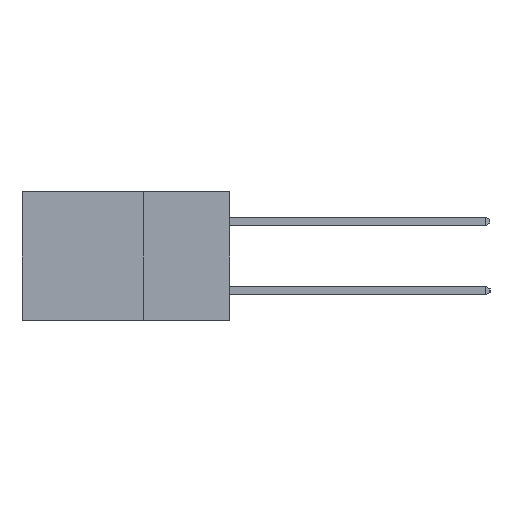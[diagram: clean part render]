
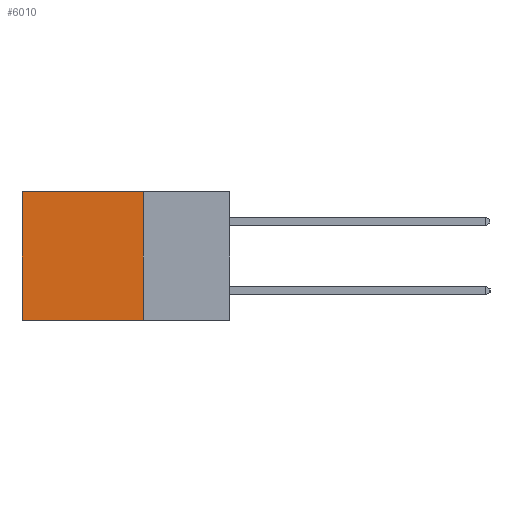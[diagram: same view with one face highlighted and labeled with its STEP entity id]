
A CAD part, left-side view. The second image highlights one B-rep face of the part: STEP entity #6010.
In plain terms, the highlighted planar face has unit normal (-1, 0, 0).
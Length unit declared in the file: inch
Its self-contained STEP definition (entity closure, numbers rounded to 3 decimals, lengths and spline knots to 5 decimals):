
#1495 = ORIENTED_EDGE ( 'NONE', *, *, #3555, .T. ) ;
#1730 = DIRECTION ( 'NONE',  ( 0., 0., -1. ) ) ;
#1794 = CARTESIAN_POINT ( 'NONE',  ( 0.2615, 0.6, -0.37 ) ) ;
#2799 = DIRECTION ( 'NONE',  ( 0., 1., 0. ) ) ;
#2877 = CARTESIAN_POINT ( 'NONE',  ( 0.2615, 0.25, -0.37 ) ) ;
#3468 = EDGE_CURVE ( 'NONE', #6410, #3936, #7399, .T. ) ;
#3555 = EDGE_CURVE ( 'NONE', #5289, #3936, #5964, .T. ) ;
#3936 = VERTEX_POINT ( 'NONE', #13215 ) ;
#4170 = CARTESIAN_POINT ( 'NONE',  ( 0.2615, 0.25, 0. ) ) ;
#5289 = VERTEX_POINT ( 'NONE', #14054 ) ;
#5964 = LINE ( 'NONE', #1794, #14185 ) ;
#6010 = ADVANCED_FACE ( 'NONE', ( #9214 ), #10509, .F. ) ;
#6410 = VERTEX_POINT ( 'NONE', #8083 ) ;
#7280 = VERTEX_POINT ( 'NONE', #4170 ) ;
#7399 = LINE ( 'NONE', #2877, #14465 ) ;
#7968 = ORIENTED_EDGE ( 'NONE', *, *, #9770, .T. ) ;
#8083 = CARTESIAN_POINT ( 'NONE',  ( 0.2615, 0.25, -0.37 ) ) ;
#9163 = EDGE_CURVE ( 'NONE', #7280, #6410, #13386, .T. ) ;
#9214 = FACE_OUTER_BOUND ( 'NONE', #13059, .T. ) ;
#9770 = EDGE_CURVE ( 'NONE', #7280, #5289, #14300, .T. ) ;
#10238 = VECTOR ( 'NONE', #11351, 39.37008 ) ;
#10475 = DIRECTION ( 'NONE',  ( 0., 0., -1. ) ) ;
#10491 = DIRECTION ( 'NONE',  ( 1., 0., 0. ) ) ;
#10493 = CARTESIAN_POINT ( 'NONE',  ( 0.2615, 0.25, -0.37 ) ) ;
#10509 = PLANE ( 'NONE',  #11107 ) ;
#10599 = VECTOR ( 'NONE', #10788, 39.37008 ) ;
#10777 = CARTESIAN_POINT ( 'NONE',  ( 0.2615, 0.25, -0.37 ) ) ;
#10788 = DIRECTION ( 'NONE',  ( 0., 0., -1. ) ) ;
#10805 = ORIENTED_EDGE ( 'NONE', *, *, #3468, .F. ) ;
#11107 = AXIS2_PLACEMENT_3D ( 'NONE', #10493, #10491, #10475 ) ;
#11351 = DIRECTION ( 'NONE',  ( 0., 1., 0. ) ) ;
#11380 = CARTESIAN_POINT ( 'NONE',  ( 0.2615, 0.25, 0. ) ) ;
#13059 = EDGE_LOOP ( 'NONE', ( #1495, #10805, #13570, #7968 ) ) ;
#13215 = CARTESIAN_POINT ( 'NONE',  ( 0.2615, 0.6, -0.37 ) ) ;
#13386 = LINE ( 'NONE', #10777, #10599 ) ;
#13570 = ORIENTED_EDGE ( 'NONE', *, *, #9163, .F. ) ;
#14054 = CARTESIAN_POINT ( 'NONE',  ( 0.2615, 0.6, 0. ) ) ;
#14185 = VECTOR ( 'NONE', #1730, 39.37008 ) ;
#14300 = LINE ( 'NONE', #11380, #10238 ) ;
#14465 = VECTOR ( 'NONE', #2799, 39.37008 ) ;
